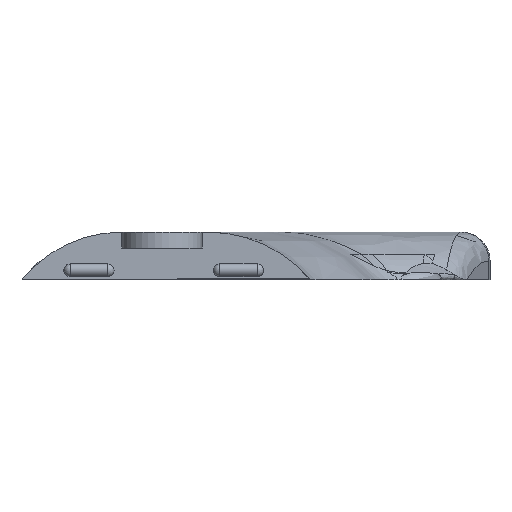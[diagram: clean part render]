
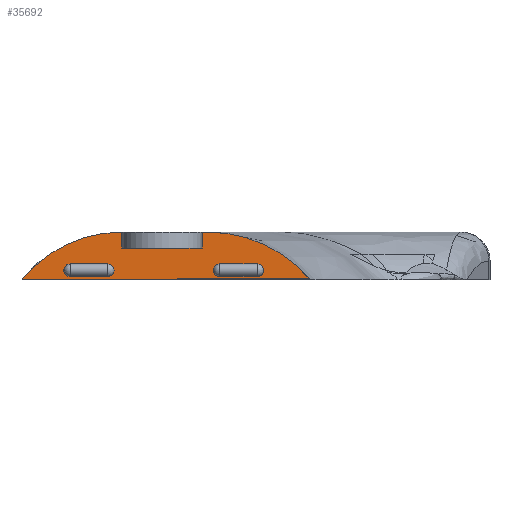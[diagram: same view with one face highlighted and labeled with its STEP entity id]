
A CAD part, front view. The second image highlights one B-rep face of the part: STEP entity #35692.
In plain terms, the highlighted planar face has unit normal (0, -1, 0).
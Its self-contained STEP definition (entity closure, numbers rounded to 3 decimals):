
#70=B_SPLINE_CURVE_WITH_KNOTS('',3,(#71272,#71273,#71274,#71275,#71276,
#71277,#71278,#71279),.UNSPECIFIED.,.F.,.F.,(4,2,2,4),(-1.806,
-1.329,-0.82,0.),.UNSPECIFIED.);
#84=B_SPLINE_CURVE_WITH_KNOTS('',3,(#71778,#71779,#71780,#71781,#71782,
#71783,#71784,#71785),.UNSPECIFIED.,.F.,.F.,(4,2,2,4),(-1.797,
-1.301,-0.806,-0.032),.UNSPECIFIED.);
#118=CIRCLE('',#36024,1.);
#122=CIRCLE('',#36031,1.);
#124=CIRCLE('',#36035,1.);
#128=CIRCLE('',#36042,1.);
#309=FACE_BOUND('',#4704,.T.);
#310=FACE_BOUND('',#4705,.T.);
#604=PLANE('',#36074);
#2567=FACE_OUTER_BOUND('',#4703,.T.);
#4703=EDGE_LOOP('',(#31956,#31957,#31958,#31959,#31960,#31961,#31962,#31963));
#4704=EDGE_LOOP('',(#31964,#31965,#31966,#31967));
#4705=EDGE_LOOP('',(#31968,#31969,#31970,#31971));
#6751=LINE('',#70743,#8829);
#6752=LINE('',#70747,#8830);
#6767=LINE('',#71034,#8845);
#6784=LINE('',#71542,#8862);
#6785=LINE('',#71544,#8863);
#6797=LINE('',#72412,#8875);
#6798=LINE('',#72414,#8876);
#6799=LINE('',#72415,#8877);
#6800=LINE('',#72416,#8878);
#6801=LINE('',#72417,#8879);
#8829=VECTOR('',#38388,10.);
#8830=VECTOR('',#38391,10.);
#8845=VECTOR('',#38754,10.);
#8862=VECTOR('',#38791,10.);
#8863=VECTOR('',#38794,10.);
#8875=VECTOR('',#38844,10.);
#8876=VECTOR('',#38845,10.);
#8877=VECTOR('',#38846,10.);
#8878=VECTOR('',#38847,10.);
#8879=VECTOR('',#38848,10.);
#15683=VERTEX_POINT('',#70728);
#15684=VERTEX_POINT('',#70742);
#15685=VERTEX_POINT('',#70744);
#15686=VERTEX_POINT('',#70746);
#15693=VERTEX_POINT('',#70968);
#15694=VERTEX_POINT('',#70970);
#15697=VERTEX_POINT('',#70983);
#15698=VERTEX_POINT('',#70985);
#15701=VERTEX_POINT('',#70993);
#15702=VERTEX_POINT('',#70995);
#15705=VERTEX_POINT('',#71008);
#15706=VERTEX_POINT('',#71010);
#15708=VERTEX_POINT('',#71016);
#15709=VERTEX_POINT('',#71033);
#15765=VERTEX_POINT('',#72411);
#15766=VERTEX_POINT('',#72413);
#21067=EDGE_CURVE('',#15683,#15684,#6751,.F.);
#21069=EDGE_CURVE('',#15685,#15686,#6752,.F.);
#21077=EDGE_CURVE('',#15693,#15694,#118,.F.);
#21085=EDGE_CURVE('',#15697,#15698,#122,.F.);
#21089=EDGE_CURVE('',#15701,#15702,#124,.F.);
#21097=EDGE_CURVE('',#15705,#15706,#128,.F.);
#21100=EDGE_CURVE('',#15708,#15709,#6767,.T.);
#21109=EDGE_CURVE('',#15686,#15708,#70,.F.);
#21138=EDGE_CURVE('',#15706,#15701,#6784,.T.);
#21139=EDGE_CURVE('',#15698,#15693,#6785,.T.);
#21151=EDGE_CURVE('',#15709,#15683,#84,.F.);
#21181=EDGE_CURVE('',#15765,#15685,#6797,.F.);
#21182=EDGE_CURVE('',#15766,#15765,#6798,.F.);
#21183=EDGE_CURVE('',#15766,#15684,#6799,.T.);
#21184=EDGE_CURVE('',#15694,#15697,#6800,.T.);
#21185=EDGE_CURVE('',#15702,#15705,#6801,.T.);
#31956=ORIENTED_EDGE('',*,*,#21100,.F.);
#31957=ORIENTED_EDGE('',*,*,#21109,.F.);
#31958=ORIENTED_EDGE('',*,*,#21069,.F.);
#31959=ORIENTED_EDGE('',*,*,#21181,.F.);
#31960=ORIENTED_EDGE('',*,*,#21182,.F.);
#31961=ORIENTED_EDGE('',*,*,#21183,.T.);
#31962=ORIENTED_EDGE('',*,*,#21067,.F.);
#31963=ORIENTED_EDGE('',*,*,#21151,.F.);
#31964=ORIENTED_EDGE('',*,*,#21139,.F.);
#31965=ORIENTED_EDGE('',*,*,#21085,.F.);
#31966=ORIENTED_EDGE('',*,*,#21184,.F.);
#31967=ORIENTED_EDGE('',*,*,#21077,.F.);
#31968=ORIENTED_EDGE('',*,*,#21138,.F.);
#31969=ORIENTED_EDGE('',*,*,#21097,.F.);
#31970=ORIENTED_EDGE('',*,*,#21185,.F.);
#31971=ORIENTED_EDGE('',*,*,#21089,.F.);
#35692=ADVANCED_FACE('',(#2567,#309,#310),#604,.T.);
#36024=AXIS2_PLACEMENT_3D('',#70971,#38701,#38702);
#36031=AXIS2_PLACEMENT_3D('',#70986,#38719,#38720);
#36035=AXIS2_PLACEMENT_3D('',#70996,#38729,#38730);
#36042=AXIS2_PLACEMENT_3D('',#71011,#38747,#38748);
#36074=AXIS2_PLACEMENT_3D('',#72410,#38842,#38843);
#38388=DIRECTION('',(-1.,0.,0.));
#38391=DIRECTION('',(-1.,0.,0.));
#38701=DIRECTION('center_axis',(0.,1.,0.));
#38702=DIRECTION('ref_axis',(-0.707,0.,0.707));
#38719=DIRECTION('center_axis',(0.,1.,0.));
#38720=DIRECTION('ref_axis',(0.707,0.,-0.707));
#38729=DIRECTION('center_axis',(0.,1.,0.));
#38730=DIRECTION('ref_axis',(-0.707,0.,0.707));
#38747=DIRECTION('center_axis',(0.,1.,0.));
#38748=DIRECTION('ref_axis',(0.707,0.,-0.707));
#38754=DIRECTION('',(-1.,0.,0.));
#38791=DIRECTION('',(-1.,0.,0.));
#38794=DIRECTION('',(-1.,0.,0.));
#38842=DIRECTION('center_axis',(0.,-1.,0.));
#38843=DIRECTION('ref_axis',(1.,0.,0.));
#38844=DIRECTION('',(0.,0.,-1.));
#38845=DIRECTION('',(-1.,0.,0.));
#38846=DIRECTION('',(0.,0.,1.));
#38847=DIRECTION('',(1.,0.,0.));
#38848=DIRECTION('',(1.,0.,0.));
#70728=CARTESIAN_POINT('',(-58.318,-39.3,35.));
#70742=CARTESIAN_POINT('',(-58.256,-39.3,35.));
#70743=CARTESIAN_POINT('',(-36.678,-39.3,35.));
#70744=CARTESIAN_POINT('',(-45.656,-39.3,35.));
#70746=CARTESIAN_POINT('',(-44.729,-39.3,35.));
#70747=CARTESIAN_POINT('',(-36.678,-39.3,35.));
#70968=CARTESIAN_POINT('',(-42.884,-39.3,30.));
#70970=CARTESIAN_POINT('',(-42.884,-39.3,28.));
#70971=CARTESIAN_POINT('Origin',(-42.884,-39.3,29.));
#70983=CARTESIAN_POINT('',(-36.984,-39.3,28.));
#70985=CARTESIAN_POINT('',(-36.984,-39.3,30.));
#70986=CARTESIAN_POINT('Origin',(-36.984,-39.3,29.));
#70993=CARTESIAN_POINT('',(-66.384,-39.3,30.));
#70995=CARTESIAN_POINT('',(-66.384,-39.3,28.));
#70996=CARTESIAN_POINT('Origin',(-66.384,-39.3,29.));
#71008=CARTESIAN_POINT('',(-60.484,-39.3,28.));
#71010=CARTESIAN_POINT('',(-60.484,-39.3,30.));
#71011=CARTESIAN_POINT('Origin',(-60.484,-39.3,29.));
#71016=CARTESIAN_POINT('',(-28.831,-39.3,27.75));
#71033=CARTESIAN_POINT('',(-73.953,-39.3,27.5));
#71034=CARTESIAN_POINT('',(-39.44,-39.3,27.75));
#71272=CARTESIAN_POINT('Ctrl Pts',(-28.831,-39.3,
27.75));
#71273=CARTESIAN_POINT('Ctrl Pts',(-29.872,-39.3,
28.949));
#71274=CARTESIAN_POINT('Ctrl Pts',(-31.045,-39.3,
30.027));
#71275=CARTESIAN_POINT('Ctrl Pts',(-33.699,-39.3,31.961));
#71276=CARTESIAN_POINT('Ctrl Pts',(-35.185,-39.3,32.79));
#71277=CARTESIAN_POINT('Ctrl Pts',(-39.286,-39.3,
34.468));
#71278=CARTESIAN_POINT('Ctrl Pts',(-41.994,-39.3,35.));
#71279=CARTESIAN_POINT('Ctrl Pts',(-44.729,-39.3,
35.));
#71542=CARTESIAN_POINT('',(-39.44,-39.3,30.));
#71544=CARTESIAN_POINT('',(-39.44,-39.3,30.));
#71778=CARTESIAN_POINT('Ctrl Pts',(-58.318,-39.3,
35.));
#71779=CARTESIAN_POINT('Ctrl Pts',(-59.971,-39.3,
35.));
#71780=CARTESIAN_POINT('Ctrl Pts',(-61.618,-39.3,
34.796));
#71781=CARTESIAN_POINT('Ctrl Pts',(-64.822,-39.3,33.989));
#71782=CARTESIAN_POINT('Ctrl Pts',(-66.367,-39.3,
33.389));
#71783=CARTESIAN_POINT('Ctrl Pts',(-70.092,-39.3,
31.384));
#71784=CARTESIAN_POINT('Ctrl Pts',(-72.105,-39.3,
29.735));
#71785=CARTESIAN_POINT('Ctrl Pts',(-73.749,-39.3,27.75));
#72410=CARTESIAN_POINT('Origin',(-36.184,-39.3,27.5));
#72411=CARTESIAN_POINT('',(-45.656,-39.3,32.5));
#72412=CARTESIAN_POINT('',(-45.656,-39.3,30.));
#72413=CARTESIAN_POINT('',(-58.256,-39.3,32.5));
#72414=CARTESIAN_POINT('',(-44.07,-39.3,32.5));
#72415=CARTESIAN_POINT('',(-58.256,-39.3,32.));
#72416=CARTESIAN_POINT('',(-36.678,-39.3,28.));
#72417=CARTESIAN_POINT('',(-36.678,-39.3,28.));
